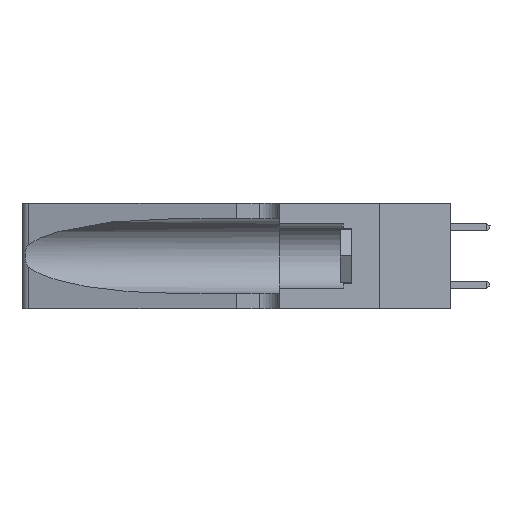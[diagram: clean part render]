
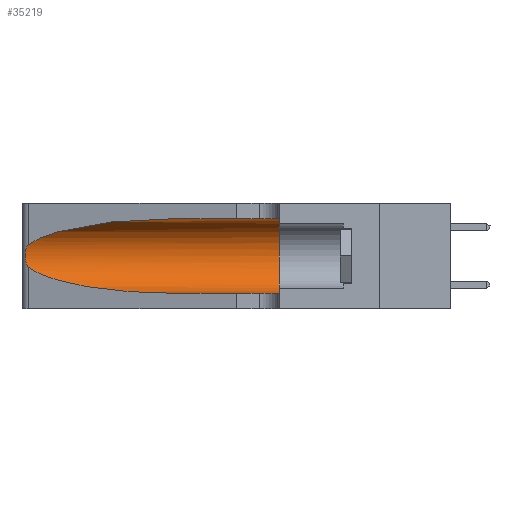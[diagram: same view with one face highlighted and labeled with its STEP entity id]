
A CAD part, left-side view. The second image highlights one B-rep face of the part: STEP entity #35219.
In plain terms, the highlighted cylindrical face has radius 3.308 mm (diameter 6.617 mm), a partial arc.
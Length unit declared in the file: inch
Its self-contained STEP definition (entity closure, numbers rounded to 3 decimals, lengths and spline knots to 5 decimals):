
#632 = CARTESIAN_POINT ( 'NONE',  ( 0.18966, 0.96281, 0.31525 ) ) ;
#708 = CARTESIAN_POINT ( 'NONE',  ( 0.1305, 0.35, 0.05475 ) ) ;
#1008 = CARTESIAN_POINT ( 'NONE',  ( 0.26075, 1.23896, 0.178 ) ) ;
#4036 = CARTESIAN_POINT ( 'NONE',  ( 0.25555, 1.22994, 0.2215 ) ) ;
#4171 = CARTESIAN_POINT ( 'NONE',  ( 0.25856, 1.23593, 0.16098 ) ) ;
#4492 = CARTESIAN_POINT ( 'NONE',  ( 0.1305, 0.72297, 0.05475 ) ) ;
#4783 = VERTEX_POINT ( 'NONE', #6828 ) ;
#5665 = CARTESIAN_POINT ( 'NONE',  ( 0.25487, 1.22718, 0.22369 ) ) ;
#6828 = CARTESIAN_POINT ( 'NONE',  ( 0.1305, 0.72297, 0.05475 ) ) ;
#6918 = LINE ( 'NONE', #29325, #37113 ) ;
#7365 = CARTESIAN_POINT ( 'NONE',  ( 0.25639, 1.23186, 0.15144 ) ) ;
#10155 = CARTESIAN_POINT ( 'NONE',  ( 0.25487, 1.22718, 0.22369 ) ) ;
#10534 = VERTEX_POINT ( 'NONE', #22371 ) ;
#10542 = CARTESIAN_POINT ( 'NONE',  ( 0.25487, 1.22718, 0.14631 ) ) ;
#12001 = EDGE_LOOP ( 'NONE', ( #39853, #18205, #15262, #37720, #13661, #13063 ) ) ;
#12240 = CIRCLE ( 'NONE', #24418, 0.13025 ) ;
#13063 = ORIENTED_EDGE ( 'NONE', *, *, #16582, .F. ) ;
#13546 = CARTESIAN_POINT ( 'NONE',  ( 0.25487, 1.22718, 0.22369 ) ) ;
#13656 = VERTEX_POINT ( 'NONE', #14538 ) ;
#13661 = ORIENTED_EDGE ( 'NONE', *, *, #17466, .F. ) ;
#14538 = CARTESIAN_POINT ( 'NONE',  ( 0.1305, 0.72297, 0.31525 ) ) ;
#15205 = EDGE_CURVE ( 'NONE', #4783, #29048, #39444, .T. ) ;
#15262 = ORIENTED_EDGE ( 'NONE', *, *, #27988, .T. ) ;
#16582 = EDGE_CURVE ( 'NONE', #13656, #10534, #6918, .T. ) ;
#16697 = CARTESIAN_POINT ( 'NONE',  ( 0.25854, 1.2359, 0.20912 ) ) ;
#16770 = CARTESIAN_POINT ( 'NONE',  ( 0.1305, 0.35, 0.185 ) ) ;
#17131 = DIRECTION ( 'NONE',  ( 0., 0., -1. ) ) ;
#17466 = EDGE_CURVE ( 'NONE', #10534, #29048, #12240, .T. ) ;
#18205 = ORIENTED_EDGE ( 'NONE', *, *, #20081, .T. ) ;
#18682 =( BOUNDED_CURVE ( )  B_SPLINE_CURVE ( 3, ( #35611, #19986, #23249, #4492 ),
 .UNSPECIFIED., .F., .F. ) 
 B_SPLINE_CURVE_WITH_KNOTS ( ( 4, 4 ),
 ( 3.44316, 4.71239 ),
 .UNSPECIFIED. ) 
 CURVE ( )  GEOMETRIC_REPRESENTATION_ITEM ( )  RATIONAL_B_SPLINE_CURVE ( ( 1., 0.87, 0.87, 1. ) ) 
 REPRESENTATION_ITEM ( '' )  );
#19802 = CARTESIAN_POINT ( 'NONE',  ( 0.26075, 1.23896, 0.19203 ) ) ;
#19880 = DIRECTION ( 'NONE',  ( 0., 0., 1. ) ) ;
#19960 = DIRECTION ( 'NONE',  ( 0., -1., 0. ) ) ;
#19986 = CARTESIAN_POINT ( 'NONE',  ( 0.2373, 1.15595, 0.08982 ) ) ;
#20081 = EDGE_CURVE ( 'NONE', #20390, #35556, #37320, .T. ) ;
#20390 = VERTEX_POINT ( 'NONE', #5665 ) ;
#21217 = EDGE_CURVE ( 'NONE', #13656, #20390, #25889, .T. ) ;
#22371 = CARTESIAN_POINT ( 'NONE',  ( 0.1305, 0.35, 0.31525 ) ) ;
#22942 = CARTESIAN_POINT ( 'NONE',  ( 0.26017, 1.23833, 0.17102 ) ) ;
#23249 = CARTESIAN_POINT ( 'NONE',  ( 0.18966, 0.96281, 0.05475 ) ) ;
#24418 = AXIS2_PLACEMENT_3D ( 'NONE', #16770, #38454, #19880 ) ;
#24824 = CARTESIAN_POINT ( 'NONE',  ( 0.25487, 1.22718, 0.14631 ) ) ;
#25669 = CARTESIAN_POINT ( 'NONE',  ( 0.1305, 0.72297, 0.31525 ) ) ;
#25889 =( BOUNDED_CURVE ( )  B_SPLINE_CURVE ( 3, ( #25669, #632, #28797, #10155 ),
 .UNSPECIFIED., .F., .T. ) 
 B_SPLINE_CURVE_WITH_KNOTS ( ( 4, 4 ),
 ( 1.5708, 2.84003 ),
 .UNSPECIFIED. ) 
 CURVE ( )  GEOMETRIC_REPRESENTATION_ITEM ( )  RATIONAL_B_SPLINE_CURVE ( ( 1., 0.87, 0.87, 1. ) ) 
 REPRESENTATION_ITEM ( '' )  );
#25921 = CARTESIAN_POINT ( 'NONE',  ( 0.25639, 1.23184, 0.21858 ) ) ;
#26062 = CARTESIAN_POINT ( 'NONE',  ( 0.25789, 1.23486, 0.15765 ) ) ;
#26172 = CARTESIAN_POINT ( 'NONE',  ( 0.1305, 1.61858, 0.05475 ) ) ;
#27988 = EDGE_CURVE ( 'NONE', #35556, #4783, #18682, .T. ) ;
#28797 = CARTESIAN_POINT ( 'NONE',  ( 0.2373, 1.15595, 0.28018 ) ) ;
#29048 = VERTEX_POINT ( 'NONE', #708 ) ;
#29176 = CARTESIAN_POINT ( 'NONE',  ( 0.25555, 1.22993, 0.14849 ) ) ;
#29325 = CARTESIAN_POINT ( 'NONE',  ( 0.1305, 1.61858, 0.31525 ) ) ;
#31234 = VECTOR ( 'NONE', #35541, 39.37008 ) ;
#32654 = AXIS2_PLACEMENT_3D ( 'NONE', #35451, #35718, #17131 ) ;
#35219 = ADVANCED_FACE ( 'NONE', ( #40277 ), #39332, .F. ) ;
#35298 = CARTESIAN_POINT ( 'NONE',  ( 0.25787, 1.23484, 0.2124 ) ) ;
#35451 = CARTESIAN_POINT ( 'NONE',  ( 0.1305, 1.61858, 0.185 ) ) ;
#35541 = DIRECTION ( 'NONE',  ( 0., -1., 0. ) ) ;
#35556 = VERTEX_POINT ( 'NONE', #24824 ) ;
#35611 = CARTESIAN_POINT ( 'NONE',  ( 0.25487, 1.22718, 0.14631 ) ) ;
#35718 = DIRECTION ( 'NONE',  ( 0., -1., 0. ) ) ;
#37113 = VECTOR ( 'NONE', #19960, 39.37008 ) ;
#37320 = B_SPLINE_CURVE_WITH_KNOTS ( 'NONE', 3,
 ( #13546, #4036, #25921, #35298, #16697, #38367, #19802, #1008, #22942, #4171, #26062, #7365, #29176, #10542 ),
 .UNSPECIFIED., .F., .F.,
 ( 4, 2, 2, 2, 2, 2, 4 ),
 ( 0., 0.00027, 0.00053, 0.00107, 0.0016, 0.00187, 0.00214 ),
 .UNSPECIFIED. ) ;
#37720 = ORIENTED_EDGE ( 'NONE', *, *, #15205, .T. ) ;
#38367 = CARTESIAN_POINT ( 'NONE',  ( 0.26018, 1.23835, 0.19895 ) ) ;
#38454 = DIRECTION ( 'NONE',  ( 0., 1., 0. ) ) ;
#39332 = CYLINDRICAL_SURFACE ( 'NONE', #32654, 0.13025 ) ;
#39444 = LINE ( 'NONE', #26172, #31234 ) ;
#39853 = ORIENTED_EDGE ( 'NONE', *, *, #21217, .T. ) ;
#40277 = FACE_OUTER_BOUND ( 'NONE', #12001, .T. ) ;
